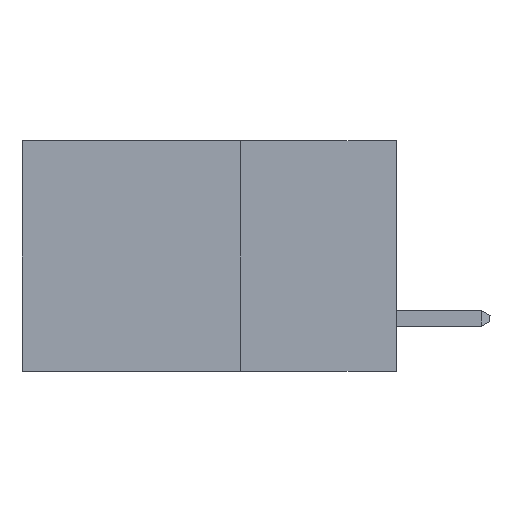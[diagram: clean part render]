
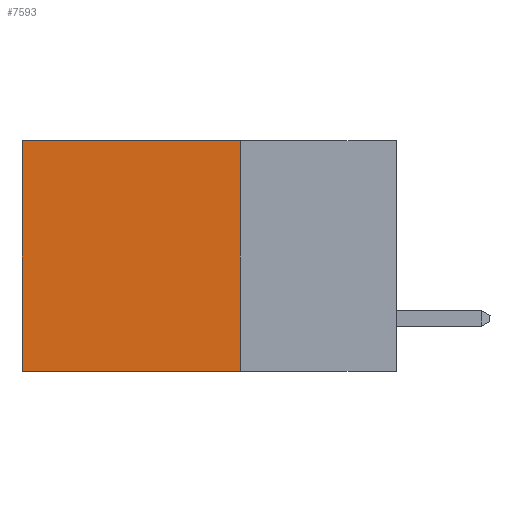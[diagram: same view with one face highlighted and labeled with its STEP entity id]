
A CAD part, left-side view. The second image highlights one B-rep face of the part: STEP entity #7593.
In plain terms, the highlighted planar face has unit normal (-1, 0, 0).
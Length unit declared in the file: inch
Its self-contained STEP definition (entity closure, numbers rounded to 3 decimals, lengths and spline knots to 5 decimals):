
#221 = EDGE_LOOP ( 'NONE', ( #13425, #492, #8843, #9708 ) ) ;
#492 = ORIENTED_EDGE ( 'NONE', *, *, #13646, .F. ) ;
#923 = VECTOR ( 'NONE', #12889, 39.37008 ) ;
#1511 = FACE_OUTER_BOUND ( 'NONE', #221, .T. ) ;
#1636 = VERTEX_POINT ( 'NONE', #5169 ) ;
#2338 = PLANE ( 'NONE',  #3632 ) ;
#2346 = LINE ( 'NONE', #10577, #9066 ) ;
#3069 = DIRECTION ( 'NONE',  ( 0., 0., -1. ) ) ;
#3157 = VERTEX_POINT ( 'NONE', #3194 ) ;
#3194 = CARTESIAN_POINT ( 'NONE',  ( 0.2615, 0.6, -0.37 ) ) ;
#3632 = AXIS2_PLACEMENT_3D ( 'NONE', #12371, #4869, #13633 ) ;
#4133 = CARTESIAN_POINT ( 'NONE',  ( 0.2615, 0.25, 0. ) ) ;
#4869 = DIRECTION ( 'NONE',  ( 1., 0., 0. ) ) ;
#5021 = DIRECTION ( 'NONE',  ( 0., 0., -1. ) ) ;
#5169 = CARTESIAN_POINT ( 'NONE',  ( 0.2615, 0.25, -0.37 ) ) ;
#7298 = CARTESIAN_POINT ( 'NONE',  ( 0.2615, 0.6, 0. ) ) ;
#7593 = ADVANCED_FACE ( 'NONE', ( #1511 ), #2338, .F. ) ;
#8233 = EDGE_CURVE ( 'NONE', #9560, #3157, #11709, .T. ) ;
#8843 = ORIENTED_EDGE ( 'NONE', *, *, #15331, .F. ) ;
#9066 = VECTOR ( 'NONE', #3069, 39.37008 ) ;
#9560 = VERTEX_POINT ( 'NONE', #7298 ) ;
#9708 = ORIENTED_EDGE ( 'NONE', *, *, #14610, .T. ) ;
#10577 = CARTESIAN_POINT ( 'NONE',  ( 0.2615, 0.25, -0.37 ) ) ;
#10646 = CARTESIAN_POINT ( 'NONE',  ( 0.2615, 0.25, 0. ) ) ;
#10690 = VERTEX_POINT ( 'NONE', #10646 ) ;
#11709 = LINE ( 'NONE', #13765, #14608 ) ;
#12200 = VECTOR ( 'NONE', #15299, 39.37008 ) ;
#12371 = CARTESIAN_POINT ( 'NONE',  ( 0.2615, 0.25, -0.37 ) ) ;
#12889 = DIRECTION ( 'NONE',  ( 0., 1., 0. ) ) ;
#13425 = ORIENTED_EDGE ( 'NONE', *, *, #8233, .T. ) ;
#13633 = DIRECTION ( 'NONE',  ( 0., 0., -1. ) ) ;
#13646 = EDGE_CURVE ( 'NONE', #1636, #3157, #15460, .T. ) ;
#13765 = CARTESIAN_POINT ( 'NONE',  ( 0.2615, 0.6, -0.37 ) ) ;
#14078 = CARTESIAN_POINT ( 'NONE',  ( 0.2615, 0.25, -0.37 ) ) ;
#14305 = LINE ( 'NONE', #4133, #923 ) ;
#14608 = VECTOR ( 'NONE', #5021, 39.37008 ) ;
#14610 = EDGE_CURVE ( 'NONE', #10690, #9560, #14305, .T. ) ;
#15299 = DIRECTION ( 'NONE',  ( 0., 1., 0. ) ) ;
#15331 = EDGE_CURVE ( 'NONE', #10690, #1636, #2346, .T. ) ;
#15460 = LINE ( 'NONE', #14078, #12200 ) ;
